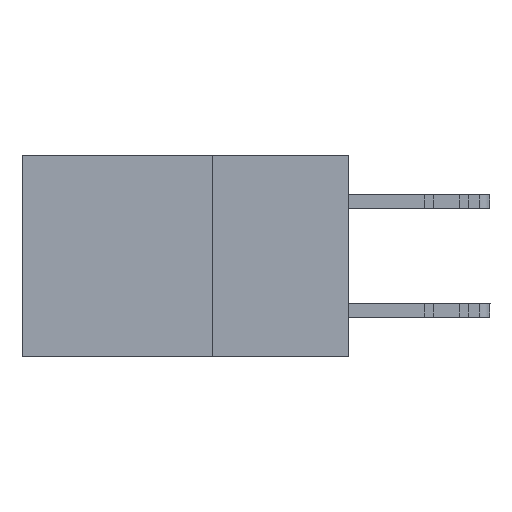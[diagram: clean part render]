
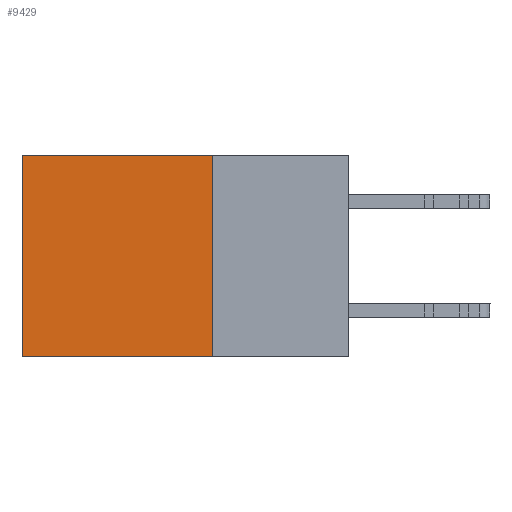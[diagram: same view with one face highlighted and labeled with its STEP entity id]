
A CAD part, left-side view. The second image highlights one B-rep face of the part: STEP entity #9429.
In plain terms, the highlighted planar face has unit normal (-1, 0, 0).
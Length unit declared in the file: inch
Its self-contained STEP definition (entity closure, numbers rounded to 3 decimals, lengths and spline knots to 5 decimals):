
#1147 = ORIENTED_EDGE ( 'NONE', *, *, #17574, .F. ) ;
#2315 = PLANE ( 'NONE',  #29992 ) ;
#2789 = VERTEX_POINT ( 'NONE', #6891 ) ;
#4823 = VECTOR ( 'NONE', #6978, 39.37008 ) ;
#6251 = LINE ( 'NONE', #11076, #26886 ) ;
#6891 = CARTESIAN_POINT ( 'NONE',  ( 0.298, 0.25, -0.37 ) ) ;
#6978 = DIRECTION ( 'NONE',  ( 0., 1., 0. ) ) ;
#7013 = DIRECTION ( 'NONE',  ( 1., 0., 0. ) ) ;
#9386 = CARTESIAN_POINT ( 'NONE',  ( 0.298, 0.6, 0. ) ) ;
#9396 = ORIENTED_EDGE ( 'NONE', *, *, #27785, .T. ) ;
#9429 = ADVANCED_FACE ( 'NONE', ( #10744 ), #2315, .F. ) ;
#10744 = FACE_OUTER_BOUND ( 'NONE', #11302, .T. ) ;
#10755 = LINE ( 'NONE', #14100, #19893 ) ;
#10872 = ORIENTED_EDGE ( 'NONE', *, *, #23793, .F. ) ;
#11076 = CARTESIAN_POINT ( 'NONE',  ( 0.298, 0.25, 0. ) ) ;
#11130 = LINE ( 'NONE', #23721, #4823 ) ;
#11302 = EDGE_LOOP ( 'NONE', ( #9396, #10872, #1147, #13947 ) ) ;
#11987 = VECTOR ( 'NONE', #27178, 39.37008 ) ;
#12820 = VERTEX_POINT ( 'NONE', #29143 ) ;
#13464 = EDGE_CURVE ( 'NONE', #18102, #16275, #6251, .T. ) ;
#13947 = ORIENTED_EDGE ( 'NONE', *, *, #13464, .T. ) ;
#14100 = CARTESIAN_POINT ( 'NONE',  ( 0.298, 0.6, 0. ) ) ;
#15650 = DIRECTION ( 'NONE',  ( 0., 1., 0. ) ) ;
#16275 = VERTEX_POINT ( 'NONE', #9386 ) ;
#16348 = LINE ( 'NONE', #29649, #11987 ) ;
#17574 = EDGE_CURVE ( 'NONE', #18102, #2789, #16348, .T. ) ;
#18102 = VERTEX_POINT ( 'NONE', #25210 ) ;
#19893 = VECTOR ( 'NONE', #21242, 39.37008 ) ;
#21242 = DIRECTION ( 'NONE',  ( 0., 0., -1. ) ) ;
#23041 = CARTESIAN_POINT ( 'NONE',  ( 0.298, 0.25, 0. ) ) ;
#23721 = CARTESIAN_POINT ( 'NONE',  ( 0.298, 0.25, -0.37 ) ) ;
#23793 = EDGE_CURVE ( 'NONE', #2789, #12820, #11130, .T. ) ;
#25210 = CARTESIAN_POINT ( 'NONE',  ( 0.298, 0.25, 0. ) ) ;
#26886 = VECTOR ( 'NONE', #15650, 39.37008 ) ;
#27178 = DIRECTION ( 'NONE',  ( 0., 0., -1. ) ) ;
#27785 = EDGE_CURVE ( 'NONE', #16275, #12820, #10755, .T. ) ;
#28031 = DIRECTION ( 'NONE',  ( 0., 0., -1. ) ) ;
#29143 = CARTESIAN_POINT ( 'NONE',  ( 0.298, 0.6, -0.37 ) ) ;
#29649 = CARTESIAN_POINT ( 'NONE',  ( 0.298, 0.25, 0. ) ) ;
#29992 = AXIS2_PLACEMENT_3D ( 'NONE', #23041, #7013, #28031 ) ;
